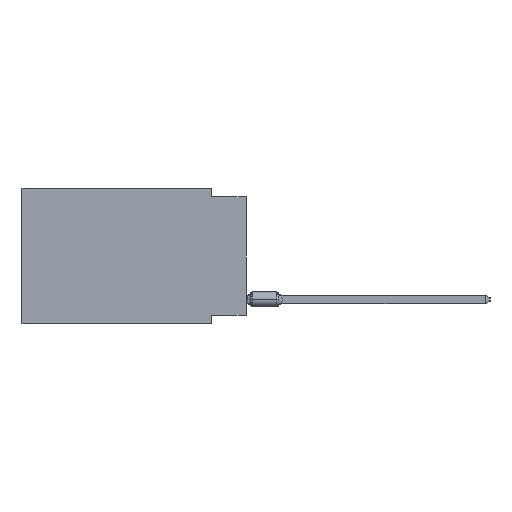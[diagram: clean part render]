
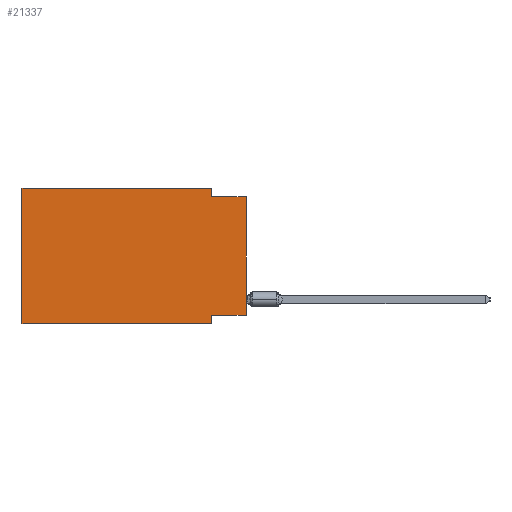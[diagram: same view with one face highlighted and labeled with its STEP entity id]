
A CAD part, left-side view. The second image highlights one B-rep face of the part: STEP entity #21337.
In plain terms, the highlighted planar face has unit normal (-1, 0, 0).
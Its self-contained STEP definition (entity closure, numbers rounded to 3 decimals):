
#279 = ORIENTED_EDGE ( 'NONE', *, *, #15361, .T. ) ;
#684 = CARTESIAN_POINT ( 'NONE',  ( 0., 16.383, 0. ) ) ;
#1693 = LINE ( 'NONE', #684, #28543 ) ;
#2296 = DIRECTION ( 'NONE',  ( 0., 0., -1. ) ) ;
#4958 = ORIENTED_EDGE ( 'NONE', *, *, #7775, .F. ) ;
#6422 = VECTOR ( 'NONE', #20024, 1000. ) ;
#6837 = DIRECTION ( 'NONE',  ( 0., 0., 1. ) ) ;
#7775 = EDGE_CURVE ( 'NONE', #25761, #39167, #67053, .T. ) ;
#10428 = LINE ( 'NONE', #51784, #6422 ) ;
#11879 = CARTESIAN_POINT ( 'NONE',  ( 0., 2.54, 0. ) ) ;
#11935 = ORIENTED_EDGE ( 'NONE', *, *, #41197, .T. ) ;
#13237 = DIRECTION ( 'NONE',  ( 0., 0., 1. ) ) ;
#14565 = CARTESIAN_POINT ( 'NONE',  ( 0., 16.383, 0. ) ) ;
#14708 = AXIS2_PLACEMENT_3D ( 'NONE', #23476, #49783, #2296 ) ;
#15361 = EDGE_CURVE ( 'NONE', #48514, #45829, #16936, .T. ) ;
#15781 = CARTESIAN_POINT ( 'NONE',  ( 0., 2.54, 0. ) ) ;
#16936 = LINE ( 'NONE', #28176, #57879 ) ;
#18530 = CARTESIAN_POINT ( 'NONE',  ( 0., 0., -0.635 ) ) ;
#19423 = CARTESIAN_POINT ( 'NONE',  ( 0., 16.383, 0. ) ) ;
#20024 = DIRECTION ( 'NONE',  ( 0., 1., 0. ) ) ;
#20249 = DIRECTION ( 'NONE',  ( 0., 0., -1. ) ) ;
#20283 = CARTESIAN_POINT ( 'NONE',  ( 0., 0., -0.635 ) ) ;
#21337 = ADVANCED_FACE ( 'NONE', ( #43979 ), #60039, .F. ) ;
#21962 = CARTESIAN_POINT ( 'NONE',  ( 0., 2.54, -9.906 ) ) ;
#23476 = CARTESIAN_POINT ( 'NONE',  ( 0., 16.383, 0. ) ) ;
#24162 = CARTESIAN_POINT ( 'NONE',  ( 0., 0., 0. ) ) ;
#25761 = VERTEX_POINT ( 'NONE', #11879 ) ;
#28149 = VERTEX_POINT ( 'NONE', #54650 ) ;
#28176 = CARTESIAN_POINT ( 'NONE',  ( 0., 16.383, -9.906 ) ) ;
#28543 = VECTOR ( 'NONE', #6837, 1000. ) ;
#28750 = CARTESIAN_POINT ( 'NONE',  ( 0., 16.383, -9.906 ) ) ;
#29548 = VERTEX_POINT ( 'NONE', #18530 ) ;
#31399 = VECTOR ( 'NONE', #40530, 1000. ) ;
#31617 = LINE ( 'NONE', #14565, #31399 ) ;
#32059 = EDGE_LOOP ( 'NONE', ( #11935, #64270, #4958, #51183, #49779, #279, #40639, #49330 ) ) ;
#33647 = EDGE_CURVE ( 'NONE', #38886, #28149, #10428, .T. ) ;
#36318 = CARTESIAN_POINT ( 'NONE',  ( 0., 2.54, -9.906 ) ) ;
#36743 = EDGE_CURVE ( 'NONE', #48514, #47986, #1693, .T. ) ;
#38886 = VERTEX_POINT ( 'NONE', #62303 ) ;
#38904 = EDGE_CURVE ( 'NONE', #39167, #29548, #67088, .T. ) ;
#39167 = VERTEX_POINT ( 'NONE', #61893 ) ;
#39200 = LINE ( 'NONE', #24162, #63396 ) ;
#40530 = DIRECTION ( 'NONE',  ( 0., -1., 0. ) ) ;
#40639 = ORIENTED_EDGE ( 'NONE', *, *, #57589, .F. ) ;
#41197 = EDGE_CURVE ( 'NONE', #38886, #29548, #39200, .T. ) ;
#41483 = VECTOR ( 'NONE', #20249, 1000. ) ;
#42111 = LINE ( 'NONE', #21962, #57400 ) ;
#43979 = FACE_OUTER_BOUND ( 'NONE', #32059, .T. ) ;
#45829 = VERTEX_POINT ( 'NONE', #36318 ) ;
#47986 = VERTEX_POINT ( 'NONE', #19423 ) ;
#48514 = VERTEX_POINT ( 'NONE', #28750 ) ;
#49330 = ORIENTED_EDGE ( 'NONE', *, *, #33647, .F. ) ;
#49719 = EDGE_CURVE ( 'NONE', #47986, #25761, #31617, .T. ) ;
#49779 = ORIENTED_EDGE ( 'NONE', *, *, #36743, .F. ) ;
#49783 = DIRECTION ( 'NONE',  ( 1., 0., 0. ) ) ;
#51183 = ORIENTED_EDGE ( 'NONE', *, *, #49719, .F. ) ;
#51784 = CARTESIAN_POINT ( 'NONE',  ( 0., 0., -9.271 ) ) ;
#52385 = DIRECTION ( 'NONE',  ( 0., 0., -1. ) ) ;
#54505 = DIRECTION ( 'NONE',  ( 0., -1., 0. ) ) ;
#54650 = CARTESIAN_POINT ( 'NONE',  ( 0., 2.54, -9.271 ) ) ;
#57400 = VECTOR ( 'NONE', #52385, 1000. ) ;
#57589 = EDGE_CURVE ( 'NONE', #28149, #45829, #42111, .T. ) ;
#57879 = VECTOR ( 'NONE', #54505, 1000. ) ;
#60039 = PLANE ( 'NONE',  #14708 ) ;
#61893 = CARTESIAN_POINT ( 'NONE',  ( 0., 2.54, -0.635 ) ) ;
#61965 = DIRECTION ( 'NONE',  ( 0., -1., 0. ) ) ;
#61988 = VECTOR ( 'NONE', #61965, 1000. ) ;
#62303 = CARTESIAN_POINT ( 'NONE',  ( 0., 0., -9.271 ) ) ;
#63396 = VECTOR ( 'NONE', #13237, 1000. ) ;
#64270 = ORIENTED_EDGE ( 'NONE', *, *, #38904, .F. ) ;
#67053 = LINE ( 'NONE', #15781, #41483 ) ;
#67088 = LINE ( 'NONE', #20283, #61988 ) ;
